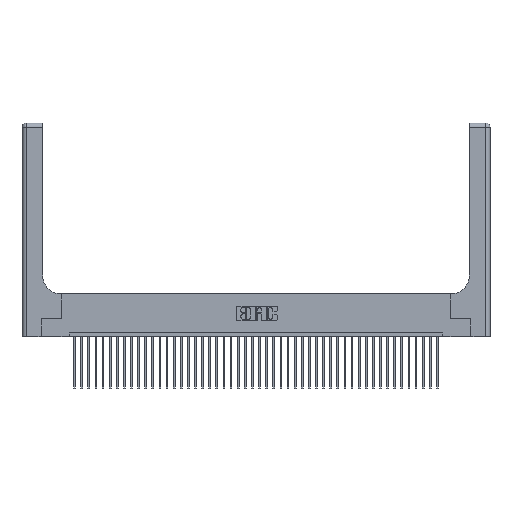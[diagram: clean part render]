
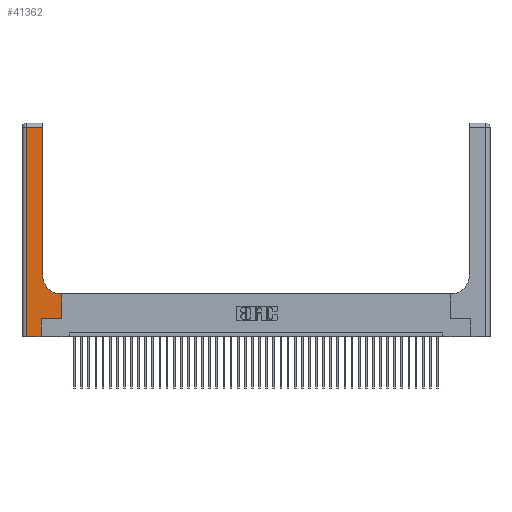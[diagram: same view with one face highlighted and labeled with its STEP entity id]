
A CAD part, top view. The second image highlights one B-rep face of the part: STEP entity #41362.
In plain terms, the highlighted planar face has unit normal (0, 0, 1).
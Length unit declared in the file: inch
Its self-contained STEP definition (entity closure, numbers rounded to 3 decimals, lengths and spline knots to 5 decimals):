
#258 = VECTOR ( 'NONE', #35999, 39.37008 ) ;
#905 = EDGE_CURVE ( 'NONE', #7330, #39988, #34371, .T. ) ;
#1337 = PLANE ( 'NONE',  #3503 ) ;
#1986 = EDGE_CURVE ( 'NONE', #16912, #35102, #21242, .T. ) ;
#2216 = VECTOR ( 'NONE', #42762, 39.37008 ) ;
#2587 = ORIENTED_EDGE ( 'NONE', *, *, #39844, .T. ) ;
#2839 = DIRECTION ( 'NONE',  ( 0., 0., -1. ) ) ;
#3416 = CARTESIAN_POINT ( 'NONE',  ( 0.5415, 0.85, 0.37 ) ) ;
#3503 = AXIS2_PLACEMENT_3D ( 'NONE', #41535, #4631, #11287 ) ;
#3537 = CARTESIAN_POINT ( 'NONE',  ( 0.2915, 2.94, 0.37 ) ) ;
#4631 = DIRECTION ( 'NONE',  ( 0., 0., -1. ) ) ;
#5963 = EDGE_CURVE ( 'NONE', #35102, #13456, #9970, .T. ) ;
#6065 = CARTESIAN_POINT ( 'NONE',  ( 0.06, 3., 0.37 ) ) ;
#6466 = LINE ( 'NONE', #8576, #42330 ) ;
#7149 = CARTESIAN_POINT ( 'NONE',  ( 0., 0., 0.37 ) ) ;
#7330 = VERTEX_POINT ( 'NONE', #3537 ) ;
#7866 = FACE_OUTER_BOUND ( 'NONE', #8498, .T. ) ;
#8498 = EDGE_LOOP ( 'NONE', ( #25088, #31816, #20551, #34817, #8570, #34777, #2587, #20111, #26907 ) ) ;
#8570 = ORIENTED_EDGE ( 'NONE', *, *, #5963, .T. ) ;
#8576 = CARTESIAN_POINT ( 'NONE',  ( 0.269, 0.25, 0.37 ) ) ;
#9401 = EDGE_CURVE ( 'NONE', #31626, #24157, #42665, .T. ) ;
#9659 = EDGE_CURVE ( 'NONE', #32660, #7330, #9956, .T. ) ;
#9956 = LINE ( 'NONE', #36040, #38563 ) ;
#9970 = LINE ( 'NONE', #19224, #2216 ) ;
#10148 = CARTESIAN_POINT ( 'NONE',  ( 0.06, 0., 0.37 ) ) ;
#11287 = DIRECTION ( 'NONE',  ( -1., 0., 0. ) ) ;
#11354 = VECTOR ( 'NONE', #33738, 39.37008 ) ;
#12346 = CARTESIAN_POINT ( 'NONE',  ( 0.06, 2.94, 0.37 ) ) ;
#12625 = LINE ( 'NONE', #41870, #33961 ) ;
#13456 = VERTEX_POINT ( 'NONE', #27852 ) ;
#13621 = CIRCLE ( 'NONE', #26689, 0.25 ) ;
#13623 = VECTOR ( 'NONE', #14825, 39.37008 ) ;
#14825 = DIRECTION ( 'NONE',  ( -1., 0., 0. ) ) ;
#16912 = VERTEX_POINT ( 'NONE', #10148 ) ;
#17746 = EDGE_CURVE ( 'NONE', #39988, #16912, #35563, .T. ) ;
#18183 = CARTESIAN_POINT ( 'NONE',  ( 0.5585, 0.6, 0.37 ) ) ;
#19224 = CARTESIAN_POINT ( 'NONE',  ( 0.269, 0., 0.37 ) ) ;
#20111 = ORIENTED_EDGE ( 'NONE', *, *, #9401, .T. ) ;
#20551 = ORIENTED_EDGE ( 'NONE', *, *, #17746, .T. ) ;
#21242 = LINE ( 'NONE', #7149, #11354 ) ;
#22900 = EDGE_CURVE ( 'NONE', #24157, #32660, #13621, .T. ) ;
#24157 = VERTEX_POINT ( 'NONE', #28754 ) ;
#25088 = ORIENTED_EDGE ( 'NONE', *, *, #9659, .T. ) ;
#25401 = CARTESIAN_POINT ( 'NONE',  ( 0.269, 0., 0.37 ) ) ;
#25701 = DIRECTION ( 'NONE',  ( 0., 1., 0. ) ) ;
#25908 = EDGE_CURVE ( 'NONE', #13456, #37958, #6466, .T. ) ;
#26537 = VECTOR ( 'NONE', #32799, 39.37008 ) ;
#26689 = AXIS2_PLACEMENT_3D ( 'NONE', #3416, #2839, #36539 ) ;
#26907 = ORIENTED_EDGE ( 'NONE', *, *, #22900, .T. ) ;
#27852 = CARTESIAN_POINT ( 'NONE',  ( 0.269, 0.25, 0.37 ) ) ;
#28754 = CARTESIAN_POINT ( 'NONE',  ( 0.5415, 0.6, 0.37 ) ) ;
#29475 = DIRECTION ( 'NONE',  ( 0., 1., 0. ) ) ;
#31439 = CARTESIAN_POINT ( 'NONE',  ( 0.5585, 0.25, 0.37 ) ) ;
#31626 = VERTEX_POINT ( 'NONE', #18183 ) ;
#31816 = ORIENTED_EDGE ( 'NONE', *, *, #905, .T. ) ;
#32504 = CARTESIAN_POINT ( 'NONE',  ( 0., 2.94, 0.37 ) ) ;
#32660 = VERTEX_POINT ( 'NONE', #42270 ) ;
#32799 = DIRECTION ( 'NONE',  ( -1., 0., 0. ) ) ;
#33738 = DIRECTION ( 'NONE',  ( 1., 0., 0. ) ) ;
#33961 = VECTOR ( 'NONE', #25701, 39.37008 ) ;
#34371 = LINE ( 'NONE', #32504, #26537 ) ;
#34757 = CARTESIAN_POINT ( 'NONE',  ( 0.2915, 0.6, 0.37 ) ) ;
#34777 = ORIENTED_EDGE ( 'NONE', *, *, #25908, .T. ) ;
#34817 = ORIENTED_EDGE ( 'NONE', *, *, #1986, .T. ) ;
#35102 = VERTEX_POINT ( 'NONE', #25401 ) ;
#35563 = LINE ( 'NONE', #6065, #258 ) ;
#35999 = DIRECTION ( 'NONE',  ( 0., -1., 0. ) ) ;
#36040 = CARTESIAN_POINT ( 'NONE',  ( 0.2915, 3., 0.37 ) ) ;
#36539 = DIRECTION ( 'NONE',  ( 1., 0., 0. ) ) ;
#37958 = VERTEX_POINT ( 'NONE', #31439 ) ;
#38563 = VECTOR ( 'NONE', #29475, 39.37008 ) ;
#39844 = EDGE_CURVE ( 'NONE', #37958, #31626, #12625, .T. ) ;
#39988 = VERTEX_POINT ( 'NONE', #12346 ) ;
#41362 = ADVANCED_FACE ( 'NONE', ( #7866 ), #1337, .F. ) ;
#41535 = CARTESIAN_POINT ( 'NONE',  ( 0., 3., 0.37 ) ) ;
#41870 = CARTESIAN_POINT ( 'NONE',  ( 0.5585, 0.25, 0.37 ) ) ;
#42003 = DIRECTION ( 'NONE',  ( 1., 0., 0. ) ) ;
#42270 = CARTESIAN_POINT ( 'NONE',  ( 0.2915, 0.85, 0.37 ) ) ;
#42330 = VECTOR ( 'NONE', #42003, 39.37008 ) ;
#42665 = LINE ( 'NONE', #34757, #13623 ) ;
#42762 = DIRECTION ( 'NONE',  ( 0., 1., 0. ) ) ;
